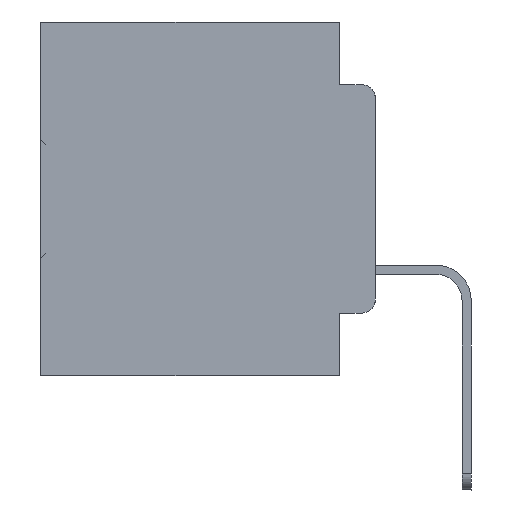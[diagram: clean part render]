
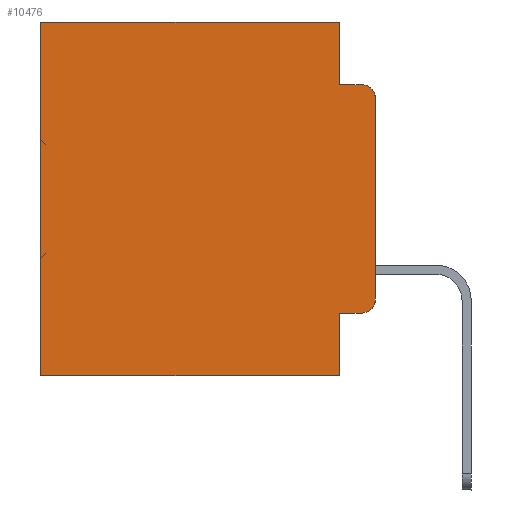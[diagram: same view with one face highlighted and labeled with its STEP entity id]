
A CAD part, left-side view. The second image highlights one B-rep face of the part: STEP entity #10476.
In plain terms, the highlighted planar face has unit normal (-1, 0, 0).
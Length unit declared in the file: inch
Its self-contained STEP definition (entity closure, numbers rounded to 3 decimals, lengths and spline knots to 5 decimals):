
#988 = AXIS2_PLACEMENT_3D ( 'NONE', #22200, #8628, #16773 ) ;
#1087 = VERTEX_POINT ( 'NONE', #27071 ) ;
#1137 = VERTEX_POINT ( 'NONE', #16181 ) ;
#1811 = ORIENTED_EDGE ( 'NONE', *, *, #35768, .T. ) ;
#1958 = ORIENTED_EDGE ( 'NONE', *, *, #9207, .F. ) ;
#2467 = EDGE_CURVE ( 'NONE', #2868, #7798, #8267, .T. ) ;
#2468 = DIRECTION ( 'NONE',  ( 0., 0., -1. ) ) ;
#2605 = VECTOR ( 'NONE', #25903, 39.37008 ) ;
#2868 = VERTEX_POINT ( 'NONE', #19363 ) ;
#3089 = EDGE_CURVE ( 'NONE', #14667, #7798, #18508, .T. ) ;
#3765 = FACE_OUTER_BOUND ( 'NONE', #24480, .T. ) ;
#4288 = LINE ( 'NONE', #27506, #18021 ) ;
#5329 = AXIS2_PLACEMENT_3D ( 'NONE', #15467, #12818, #35046 ) ;
#5709 = DIRECTION ( 'NONE',  ( 0., 0., -1. ) ) ;
#6066 = CARTESIAN_POINT ( 'NONE',  ( 0.298, 0.473, -0.5 ) ) ;
#6637 = DIRECTION ( 'NONE',  ( 0., 0., -1. ) ) ;
#6754 = EDGE_CURVE ( 'NONE', #30725, #35125, #22162, .T. ) ;
#6782 = CARTESIAN_POINT ( 'NONE',  ( 0.298, 0., -0.3915 ) ) ;
#6946 = CARTESIAN_POINT ( 'NONE',  ( 0.298, 0.473, 0. ) ) ;
#7210 = EDGE_CURVE ( 'NONE', #35125, #1087, #12256, .T. ) ;
#7706 = ORIENTED_EDGE ( 'NONE', *, *, #7210, .F. ) ;
#7798 = VERTEX_POINT ( 'NONE', #6782 ) ;
#8196 = DIRECTION ( 'NONE',  ( 0., -1., 0. ) ) ;
#8267 = CIRCLE ( 'NONE', #24323, 0.02 ) ;
#8628 = DIRECTION ( 'NONE',  ( 1., 0., 0. ) ) ;
#9207 = EDGE_CURVE ( 'NONE', #1137, #23790, #4288, .T. ) ;
#10476 = ADVANCED_FACE ( 'NONE', ( #3765 ), #22076, .F. ) ;
#10810 = ORIENTED_EDGE ( 'NONE', *, *, #14780, .T. ) ;
#12022 = ORIENTED_EDGE ( 'NONE', *, *, #15195, .T. ) ;
#12097 = ORIENTED_EDGE ( 'NONE', *, *, #3089, .F. ) ;
#12256 = LINE ( 'NONE', #17586, #17825 ) ;
#12818 = DIRECTION ( 'NONE',  ( -1., 0., 0. ) ) ;
#14098 = DIRECTION ( 'NONE',  ( 0., 1., 0. ) ) ;
#14667 = VERTEX_POINT ( 'NONE', #18618 ) ;
#14780 = EDGE_CURVE ( 'NONE', #1137, #2868, #22995, .T. ) ;
#14909 = DIRECTION ( 'NONE',  ( -1., 0., 0. ) ) ;
#15195 = EDGE_CURVE ( 'NONE', #14667, #1087, #27734, .T. ) ;
#15467 = CARTESIAN_POINT ( 'NONE',  ( 0.298, 0.02, -0.1085 ) ) ;
#16181 = CARTESIAN_POINT ( 'NONE',  ( 0.298, 0.051, -0.4115 ) ) ;
#16773 = DIRECTION ( 'NONE',  ( 0., 0., -1. ) ) ;
#17586 = CARTESIAN_POINT ( 'NONE',  ( 0.298, 0.051, -0.0885 ) ) ;
#17825 = VECTOR ( 'NONE', #20249, 39.37008 ) ;
#17931 = VECTOR ( 'NONE', #14098, 39.37008 ) ;
#18021 = VECTOR ( 'NONE', #5709, 39.37008 ) ;
#18179 = VECTOR ( 'NONE', #29923, 39.37008 ) ;
#18508 = LINE ( 'NONE', #25662, #2605 ) ;
#18618 = CARTESIAN_POINT ( 'NONE',  ( 0.298, 0., -0.1085 ) ) ;
#19363 = CARTESIAN_POINT ( 'NONE',  ( 0.298, 0.02, -0.4115 ) ) ;
#20249 = DIRECTION ( 'NONE',  ( 0., -1., 0. ) ) ;
#21365 = CARTESIAN_POINT ( 'NONE',  ( 0.298, 0.051, 0. ) ) ;
#22075 = LINE ( 'NONE', #29798, #18179 ) ;
#22076 = PLANE ( 'NONE',  #988 ) ;
#22162 = LINE ( 'NONE', #21365, #24353 ) ;
#22200 = CARTESIAN_POINT ( 'NONE',  ( 0.298, 0., 0. ) ) ;
#22995 = LINE ( 'NONE', #24542, #29511 ) ;
#23353 = CARTESIAN_POINT ( 'NONE',  ( 0.298, 0.051, -0.5 ) ) ;
#23790 = VERTEX_POINT ( 'NONE', #23353 ) ;
#24075 = VECTOR ( 'NONE', #28170, 39.37008 ) ;
#24323 = AXIS2_PLACEMENT_3D ( 'NONE', #34118, #14909, #6637 ) ;
#24353 = VECTOR ( 'NONE', #2468, 39.37008 ) ;
#24480 = EDGE_LOOP ( 'NONE', ( #12097, #12022, #7706, #26179, #1811, #34553, #27810, #1958, #10810, #28404 ) ) ;
#24542 = CARTESIAN_POINT ( 'NONE',  ( 0.298, 0.051, -0.4115 ) ) ;
#25662 = CARTESIAN_POINT ( 'NONE',  ( 0.298, 0., 0. ) ) ;
#25903 = DIRECTION ( 'NONE',  ( 0., 0., -1. ) ) ;
#26179 = ORIENTED_EDGE ( 'NONE', *, *, #6754, .F. ) ;
#26340 = CARTESIAN_POINT ( 'NONE',  ( 0.298, 0.051, 0. ) ) ;
#27071 = CARTESIAN_POINT ( 'NONE',  ( 0.298, 0.02, -0.0885 ) ) ;
#27506 = CARTESIAN_POINT ( 'NONE',  ( 0.298, 0.051, 0. ) ) ;
#27719 = VERTEX_POINT ( 'NONE', #6066 ) ;
#27734 = CIRCLE ( 'NONE', #5329, 0.02 ) ;
#27810 = ORIENTED_EDGE ( 'NONE', *, *, #34514, .F. ) ;
#28120 = EDGE_CURVE ( 'NONE', #32843, #27719, #22075, .T. ) ;
#28170 = DIRECTION ( 'NONE',  ( 0., 1., 0. ) ) ;
#28404 = ORIENTED_EDGE ( 'NONE', *, *, #2467, .T. ) ;
#28405 = CARTESIAN_POINT ( 'NONE',  ( 0.298, 0., -0.5 ) ) ;
#29511 = VECTOR ( 'NONE', #8196, 39.37008 ) ;
#29798 = CARTESIAN_POINT ( 'NONE',  ( 0.298, 0.473, 0. ) ) ;
#29923 = DIRECTION ( 'NONE',  ( 0., 0., -1. ) ) ;
#30439 = CARTESIAN_POINT ( 'NONE',  ( 0.298, 0.051, -0.0885 ) ) ;
#30494 = LINE ( 'NONE', #30640, #17931 ) ;
#30640 = CARTESIAN_POINT ( 'NONE',  ( 0.298, 0., 0. ) ) ;
#30725 = VERTEX_POINT ( 'NONE', #26340 ) ;
#32843 = VERTEX_POINT ( 'NONE', #6946 ) ;
#34118 = CARTESIAN_POINT ( 'NONE',  ( 0.298, 0.02, -0.3915 ) ) ;
#34514 = EDGE_CURVE ( 'NONE', #23790, #27719, #34919, .T. ) ;
#34553 = ORIENTED_EDGE ( 'NONE', *, *, #28120, .T. ) ;
#34919 = LINE ( 'NONE', #28405, #24075 ) ;
#35046 = DIRECTION ( 'NONE',  ( 0., 0., -1. ) ) ;
#35125 = VERTEX_POINT ( 'NONE', #30439 ) ;
#35768 = EDGE_CURVE ( 'NONE', #30725, #32843, #30494, .T. ) ;
